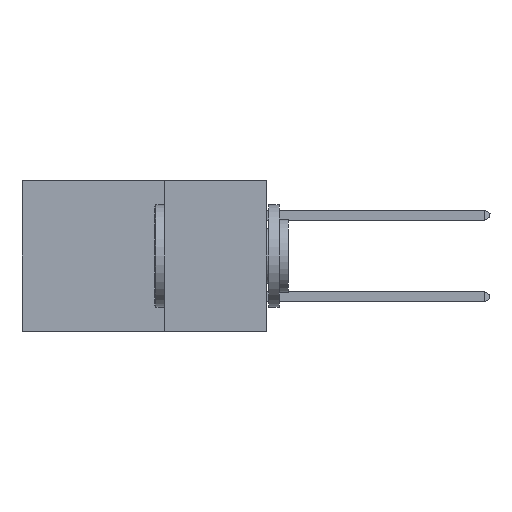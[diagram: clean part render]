
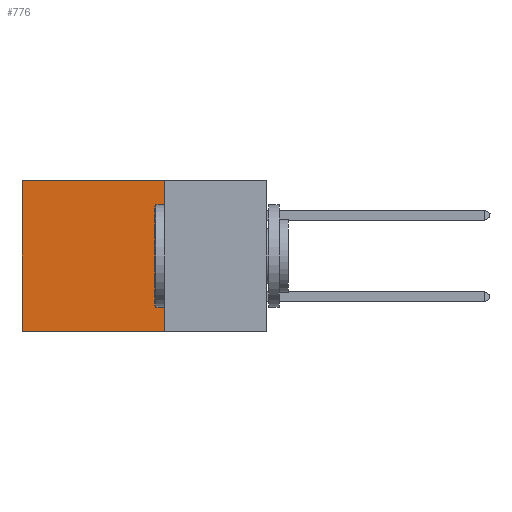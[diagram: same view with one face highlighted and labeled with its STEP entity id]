
A CAD part, left-side view. The second image highlights one B-rep face of the part: STEP entity #776.
In plain terms, the highlighted planar face has unit normal (-1, 0, 0).
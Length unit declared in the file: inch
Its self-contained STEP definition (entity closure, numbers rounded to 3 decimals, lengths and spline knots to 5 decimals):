
#290 = AXIS2_PLACEMENT_3D ( 'NONE', #1185, #1053, #10524 ) ;
#776 = ADVANCED_FACE ( 'NONE', ( #6624 ), #15931, .F. ) ;
#819 = ORIENTED_EDGE ( 'NONE', *, *, #11745, .F. ) ;
#828 = VECTOR ( 'NONE', #13798, 39.37008 ) ;
#1053 = DIRECTION ( 'NONE',  ( 1., 0., 0. ) ) ;
#1083 = LINE ( 'NONE', #12102, #10916 ) ;
#1178 = VERTEX_POINT ( 'NONE', #2904 ) ;
#1185 = CARTESIAN_POINT ( 'NONE',  ( 0.2875, 0.25, 0. ) ) ;
#1283 = LINE ( 'NONE', #2435, #12832 ) ;
#1526 = DIRECTION ( 'NONE',  ( 0., 0., -1. ) ) ;
#1934 = CARTESIAN_POINT ( 'NONE',  ( 0.2875, 0.25, -0.37 ) ) ;
#2213 = VERTEX_POINT ( 'NONE', #4487 ) ;
#2377 = EDGE_LOOP ( 'NONE', ( #5382, #8838, #819, #2822 ) ) ;
#2435 = CARTESIAN_POINT ( 'NONE',  ( 0.2875, 0.25, 0. ) ) ;
#2495 = VERTEX_POINT ( 'NONE', #4483 ) ;
#2822 = ORIENTED_EDGE ( 'NONE', *, *, #15896, .T. ) ;
#2904 = CARTESIAN_POINT ( 'NONE',  ( 0.2875, 0.6, 0. ) ) ;
#3201 = EDGE_CURVE ( 'NONE', #13572, #2495, #7106, .T. ) ;
#4483 = CARTESIAN_POINT ( 'NONE',  ( 0.2875, 0.6, -0.37 ) ) ;
#4487 = CARTESIAN_POINT ( 'NONE',  ( 0.2875, 0.25, 0. ) ) ;
#4679 = CARTESIAN_POINT ( 'NONE',  ( 0.2875, 0.25, 0. ) ) ;
#5145 = LINE ( 'NONE', #4679, #17106 ) ;
#5382 = ORIENTED_EDGE ( 'NONE', *, *, #7845, .T. ) ;
#6624 = FACE_OUTER_BOUND ( 'NONE', #2377, .T. ) ;
#7106 = LINE ( 'NONE', #11040, #828 ) ;
#7845 = EDGE_CURVE ( 'NONE', #1178, #2495, #1083, .T. ) ;
#8838 = ORIENTED_EDGE ( 'NONE', *, *, #3201, .F. ) ;
#10524 = DIRECTION ( 'NONE',  ( 0., 0., -1. ) ) ;
#10916 = VECTOR ( 'NONE', #1526, 39.37008 ) ;
#11040 = CARTESIAN_POINT ( 'NONE',  ( 0.2875, 0.25, -0.37 ) ) ;
#11745 = EDGE_CURVE ( 'NONE', #2213, #13572, #5145, .T. ) ;
#12102 = CARTESIAN_POINT ( 'NONE',  ( 0.2875, 0.6, 0. ) ) ;
#12629 = DIRECTION ( 'NONE',  ( 0., 1., 0. ) ) ;
#12832 = VECTOR ( 'NONE', #12629, 39.37008 ) ;
#13572 = VERTEX_POINT ( 'NONE', #1934 ) ;
#13798 = DIRECTION ( 'NONE',  ( 0., 1., 0. ) ) ;
#14071 = DIRECTION ( 'NONE',  ( 0., 0., -1. ) ) ;
#15896 = EDGE_CURVE ( 'NONE', #2213, #1178, #1283, .T. ) ;
#15931 = PLANE ( 'NONE',  #290 ) ;
#17106 = VECTOR ( 'NONE', #14071, 39.37008 ) ;
